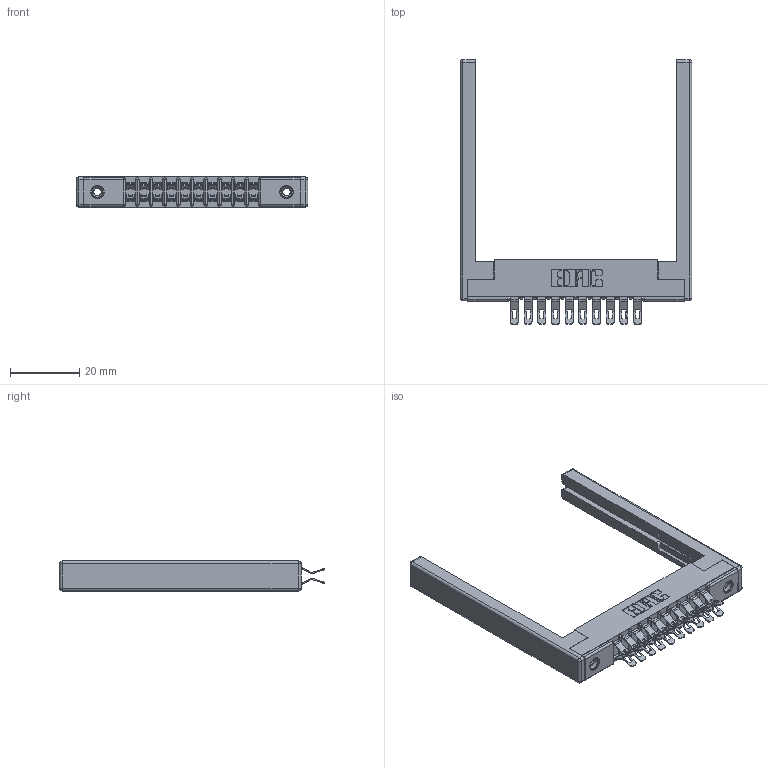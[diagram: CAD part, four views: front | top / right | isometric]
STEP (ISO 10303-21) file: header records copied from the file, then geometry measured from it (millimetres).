
FILE_DESCRIPTION (( 'STEP AP203' ), '1' );
FILE_NAME ('357-020-455-268.STEP', '2020-10-02T22:15:46', ( '' ), ( '' ), 'SwSTEP 2.0', 'SolidWorks 2020', '' );
FILE_SCHEMA (( 'CONFIG_CONTROL_DESIGN' ));
Length unit declared in the file: inch
Products named in the file (5): 345-250-001_345-250-001-102; 357-020-455-268; 307-220-068; 307-290-001_555; 307 Part_.156 Dia Mounting Holes
Assembly tree (25 placements, depth 2):
  357-020-455-268
    307 Part_.156 Dia Mounting Holes
    307-290-001_555  x20
    307-220-068  x2
    345-250-001_345-250-001-102  x2
Bounding box: 67.06 x 76.71 x 8.71 mm (x, y, z)
Volume: 9008.6 mm3; surface area: 11601.9 mm2
Topology: 25 solids, 25 shells, 1503 faces, 4333 edges, 2810 vertices
Faces by surface type: plane 838, cylinder 619, sphere 30, cone 12, torus 4
Entity records: 16134 total; most frequent: CARTESIAN_POINT 2631, DIRECTION 2613, ORIENTED_EDGE 2598, EDGE_CURVE 1299, LINE 969, VECTOR 969, VERTEX_POINT 840, AXIS2_PLACEMENT_3D 822
